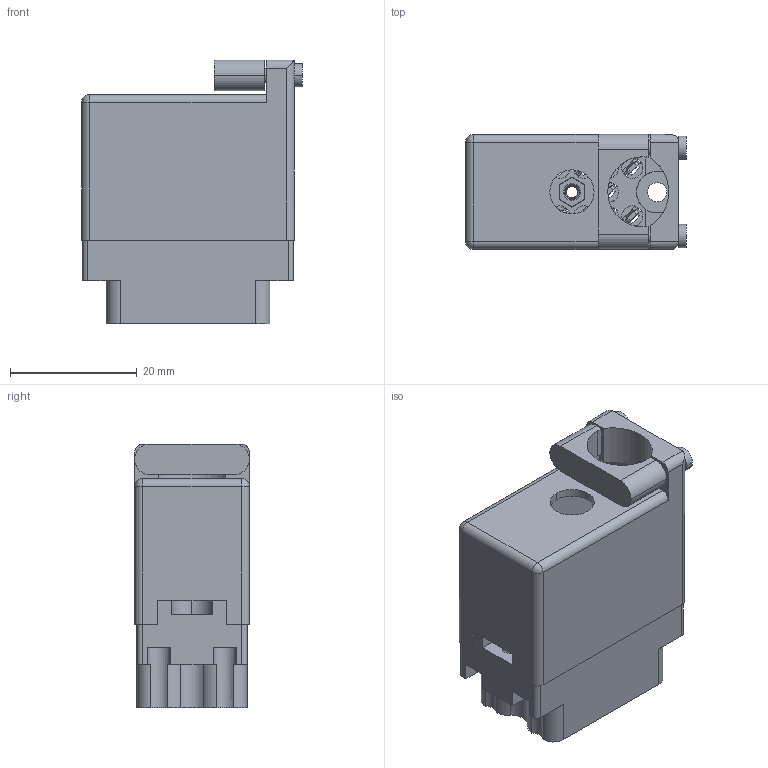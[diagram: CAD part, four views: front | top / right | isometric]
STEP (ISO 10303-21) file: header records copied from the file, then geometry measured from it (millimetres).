
FILE_DESCRIPTION (( 'STEP AP203' ), '1' );
FILE_NAME ('519-014-500-366.STEP', '2020-03-02T20:25:30', ( '' ), ( '' ), 'SwSTEP 2.0', 'SolidWorks 2016', '' );
FILE_SCHEMA (( 'CONFIG_CONTROL_DESIGN' ));
Length unit declared in the file: inch
Products named in the file (5): 516-292-001_500 Contact; 519-014-500-366; 516-252-025-100_516-252-025-100; 519 Plug Insulator_014; 516-230-001_Metal - 020 Top Entry
Assembly tree (17 placements, depth 2):
  519-014-500-366
    519 Plug Insulator_014
    516-292-001_500 Contact  x14
    516-252-025-100_516-252-025-100
    516-230-001_Metal - 020 Top Entry
Bounding box: 34.92 x 18.16 x 41.71 mm (x, y, z)
Volume: 9378.9 mm3; surface area: 14902.9 mm2
Topology: 17 solids, 17 shells, 1679 faces, 4854 edges, 3217 vertices
Faces by surface type: plane 973, cylinder 606, bspline 87, cone 11, sphere 2
Entity records: 26510 total; most frequent: CARTESIAN_POINT 7061, ORIENTED_EDGE 3984, DIRECTION 3833, EDGE_CURVE 1992, VECTOR 1363, LINE 1363, VERTEX_POINT 1319, AXIS2_PLACEMENT_3D 1235
